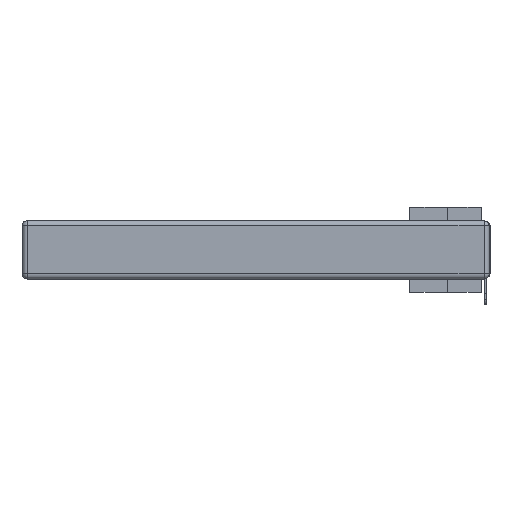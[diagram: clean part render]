
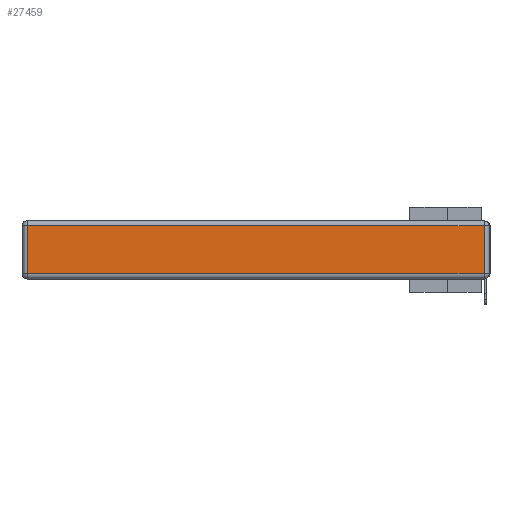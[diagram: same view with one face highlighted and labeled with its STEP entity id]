
A CAD part, left-side view. The second image highlights one B-rep face of the part: STEP entity #27459.
In plain terms, the highlighted planar face has unit normal (-1, 0, 0).
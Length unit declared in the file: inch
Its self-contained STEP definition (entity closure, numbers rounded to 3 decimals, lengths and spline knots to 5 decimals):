
#95 = VECTOR ( 'NONE', #17392, 39.37008 ) ;
#1602 = DIRECTION ( 'NONE',  ( 0., -1., 0. ) ) ;
#2422 = EDGE_CURVE ( 'NONE', #22942, #11671, #24269, .T. ) ;
#3414 = AXIS2_PLACEMENT_3D ( 'NONE', #13117, #10749, #20084 ) ;
#3700 = CARTESIAN_POINT ( 'NONE',  ( 0., 2.75, -0.03 ) ) ;
#5371 = VERTEX_POINT ( 'NONE', #28657 ) ;
#6500 = LINE ( 'NONE', #20252, #28868 ) ;
#6764 = ORIENTED_EDGE ( 'NONE', *, *, #29040, .T. ) ;
#7359 = VERTEX_POINT ( 'NONE', #22824 ) ;
#7413 = DIRECTION ( 'NONE',  ( 0., 0., -1. ) ) ;
#9222 = FACE_OUTER_BOUND ( 'NONE', #20385, .T. ) ;
#9656 = LINE ( 'NONE', #24562, #16752 ) ;
#10749 = DIRECTION ( 'NONE',  ( -1., 0., 0. ) ) ;
#11671 = VERTEX_POINT ( 'NONE', #22752 ) ;
#13117 = CARTESIAN_POINT ( 'NONE',  ( 0., 0., -0.343 ) ) ;
#13142 = ORIENTED_EDGE ( 'NONE', *, *, #18899, .T. ) ;
#16752 = VECTOR ( 'NONE', #1602, 39.37008 ) ;
#17048 = ORIENTED_EDGE ( 'NONE', *, *, #2422, .T. ) ;
#17392 = DIRECTION ( 'NONE',  ( 0., 1., 0. ) ) ;
#18899 = EDGE_CURVE ( 'NONE', #7359, #5371, #9656, .T. ) ;
#20084 = DIRECTION ( 'NONE',  ( 0., 0., 1. ) ) ;
#20088 = ORIENTED_EDGE ( 'NONE', *, *, #26219, .T. ) ;
#20252 = CARTESIAN_POINT ( 'NONE',  ( 0., 0.03, -0.343 ) ) ;
#20385 = EDGE_LOOP ( 'NONE', ( #13142, #20088, #17048, #6764 ) ) ;
#21012 = CARTESIAN_POINT ( 'NONE',  ( 0., 2.72, -0.343 ) ) ;
#22752 = CARTESIAN_POINT ( 'NONE',  ( 0., 2.72, -0.03 ) ) ;
#22824 = CARTESIAN_POINT ( 'NONE',  ( 0., 2.72, -0.313 ) ) ;
#22942 = VERTEX_POINT ( 'NONE', #29200 ) ;
#24269 = LINE ( 'NONE', #3700, #95 ) ;
#24562 = CARTESIAN_POINT ( 'NONE',  ( 0., 0., -0.313 ) ) ;
#26219 = EDGE_CURVE ( 'NONE', #5371, #22942, #6500, .T. ) ;
#26765 = PLANE ( 'NONE',  #3414 ) ;
#27124 = DIRECTION ( 'NONE',  ( 0., 0., 1. ) ) ;
#27267 = VECTOR ( 'NONE', #7413, 39.37008 ) ;
#27459 = ADVANCED_FACE ( 'NONE', ( #9222 ), #26765, .T. ) ;
#28311 = LINE ( 'NONE', #21012, #27267 ) ;
#28657 = CARTESIAN_POINT ( 'NONE',  ( 0., 0.03, -0.313 ) ) ;
#28868 = VECTOR ( 'NONE', #27124, 39.37008 ) ;
#29040 = EDGE_CURVE ( 'NONE', #11671, #7359, #28311, .T. ) ;
#29200 = CARTESIAN_POINT ( 'NONE',  ( 0., 0.03, -0.03 ) ) ;
